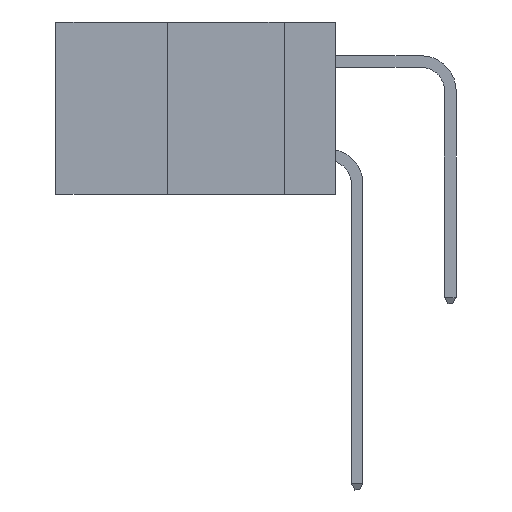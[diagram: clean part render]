
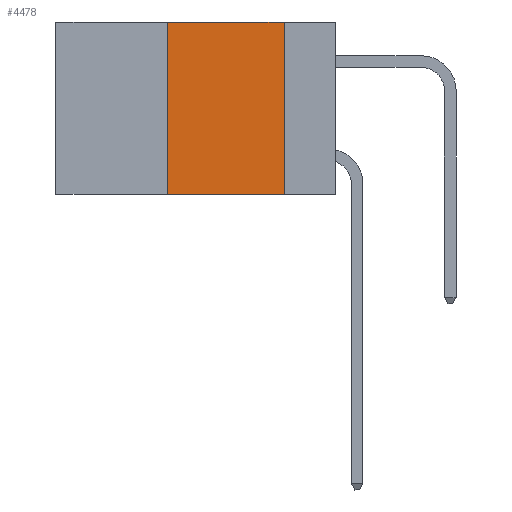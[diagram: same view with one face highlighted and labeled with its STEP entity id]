
A CAD part, left-side view. The second image highlights one B-rep face of the part: STEP entity #4478.
In plain terms, the highlighted planar face has unit normal (-1, 0, 0).
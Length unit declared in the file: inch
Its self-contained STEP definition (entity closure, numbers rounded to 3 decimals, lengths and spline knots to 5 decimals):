
#211 = AXIS2_PLACEMENT_3D ( 'NONE', #24624, #2364, #2544 ) ;
#595 = CARTESIAN_POINT ( 'NONE',  ( 0., 0.36, 0. ) ) ;
#1757 = EDGE_CURVE ( 'NONE', #3535, #19826, #9102, .T. ) ;
#2189 = PLANE ( 'NONE',  #211 ) ;
#2364 = DIRECTION ( 'NONE',  ( 1., 0., 0. ) ) ;
#2411 = EDGE_LOOP ( 'NONE', ( #9034, #12230, #22405, #8866 ) ) ;
#2544 = DIRECTION ( 'NONE',  ( 0., 0., -1. ) ) ;
#3044 = DIRECTION ( 'NONE',  ( 0., 0., 1. ) ) ;
#3535 = VERTEX_POINT ( 'NONE', #9554 ) ;
#3551 = VECTOR ( 'NONE', #23463, 39.37008 ) ;
#4193 = LINE ( 'NONE', #19654, #3551 ) ;
#4478 = ADVANCED_FACE ( 'NONE', ( #10777 ), #2189, .F. ) ;
#6041 = EDGE_CURVE ( 'NONE', #12513, #7237, #26010, .T. ) ;
#6368 = CARTESIAN_POINT ( 'NONE',  ( 0., 0.11, 0. ) ) ;
#7237 = VERTEX_POINT ( 'NONE', #595 ) ;
#8320 = DIRECTION ( 'NONE',  ( 0., 0., -1. ) ) ;
#8672 = LINE ( 'NONE', #21309, #17860 ) ;
#8866 = ORIENTED_EDGE ( 'NONE', *, *, #15428, .T. ) ;
#9034 = ORIENTED_EDGE ( 'NONE', *, *, #1757, .F. ) ;
#9102 = LINE ( 'NONE', #6368, #17978 ) ;
#9554 = CARTESIAN_POINT ( 'NONE',  ( 0., 0.11, 0. ) ) ;
#10777 = FACE_OUTER_BOUND ( 'NONE', #2411, .T. ) ;
#12230 = ORIENTED_EDGE ( 'NONE', *, *, #25025, .F. ) ;
#12513 = VERTEX_POINT ( 'NONE', #21414 ) ;
#15428 = EDGE_CURVE ( 'NONE', #12513, #19826, #8672, .T. ) ;
#16480 = VECTOR ( 'NONE', #3044, 39.37008 ) ;
#17860 = VECTOR ( 'NONE', #25572, 39.37008 ) ;
#17978 = VECTOR ( 'NONE', #8320, 39.37008 ) ;
#18162 = CARTESIAN_POINT ( 'NONE',  ( 0., 0.11, -0.37 ) ) ;
#19394 = CARTESIAN_POINT ( 'NONE',  ( 0., 0.36, 0. ) ) ;
#19654 = CARTESIAN_POINT ( 'NONE',  ( 0., 0.6, 0. ) ) ;
#19826 = VERTEX_POINT ( 'NONE', #18162 ) ;
#21309 = CARTESIAN_POINT ( 'NONE',  ( 0., 0.6, -0.37 ) ) ;
#21414 = CARTESIAN_POINT ( 'NONE',  ( 0., 0.36, -0.37 ) ) ;
#22405 = ORIENTED_EDGE ( 'NONE', *, *, #6041, .F. ) ;
#23463 = DIRECTION ( 'NONE',  ( 0., -1., 0. ) ) ;
#24624 = CARTESIAN_POINT ( 'NONE',  ( 0., 0.6, 0. ) ) ;
#25025 = EDGE_CURVE ( 'NONE', #7237, #3535, #4193, .T. ) ;
#25572 = DIRECTION ( 'NONE',  ( 0., -1., 0. ) ) ;
#26010 = LINE ( 'NONE', #19394, #16480 ) ;
